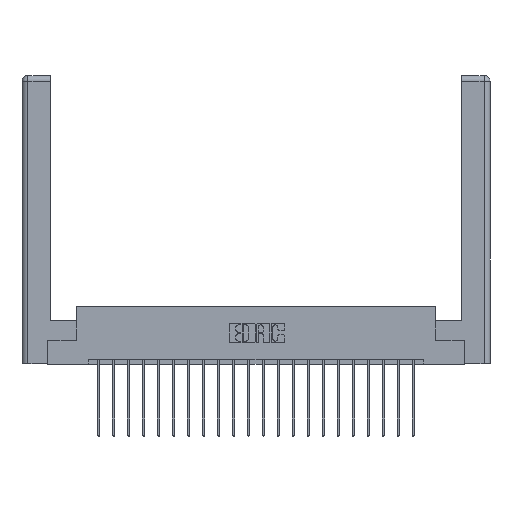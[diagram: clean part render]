
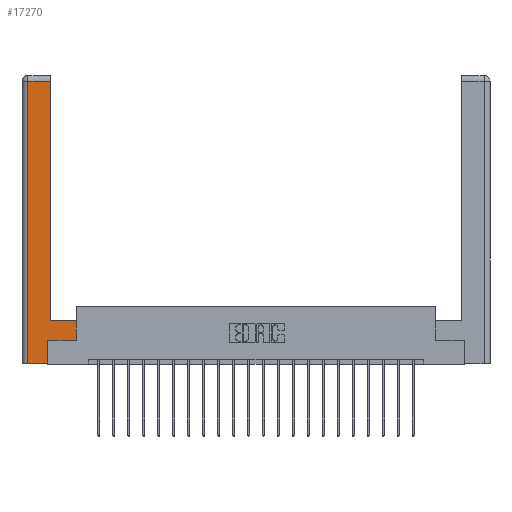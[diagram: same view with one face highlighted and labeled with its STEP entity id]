
A CAD part, top view. The second image highlights one B-rep face of the part: STEP entity #17270.
In plain terms, the highlighted planar face has unit normal (0, 0, 1).
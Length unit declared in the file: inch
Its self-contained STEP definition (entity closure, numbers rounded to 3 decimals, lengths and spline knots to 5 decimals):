
#39 = DIRECTION ( 'NONE',  ( 1., 0., 0. ) ) ;
#49 = CARTESIAN_POINT ( 'NONE',  ( 0.565, 0.245, 0. ) ) ;
#740 = DIRECTION ( 'NONE',  ( 0., 1., 0. ) ) ;
#1156 = AXIS2_PLACEMENT_3D ( 'NONE', #1345, #9943, #18810 ) ;
#1345 = CARTESIAN_POINT ( 'NONE',  ( 0., 0., 0. ) ) ;
#1348 = DIRECTION ( 'NONE',  ( 0., 1., 0. ) ) ;
#2506 = CARTESIAN_POINT ( 'NONE',  ( 0.265, 0.245, 0. ) ) ;
#2820 = EDGE_CURVE ( 'NONE', #22323, #15893, #14180, .T. ) ;
#3142 = VECTOR ( 'NONE', #3279, 39.37008 ) ;
#3279 = DIRECTION ( 'NONE',  ( 0., -1., 0. ) ) ;
#4844 = VERTEX_POINT ( 'NONE', #12020 ) ;
#5007 = CARTESIAN_POINT ( 'NONE',  ( 0.265, 0.245, 0. ) ) ;
#5040 = DIRECTION ( 'NONE',  ( -1., 0., 0. ) ) ;
#5057 = PLANE ( 'NONE',  #1156 ) ;
#5689 = EDGE_CURVE ( 'NONE', #21786, #22323, #20383, .T. ) ;
#5832 = ORIENTED_EDGE ( 'NONE', *, *, #7023, .T. ) ;
#6358 = DIRECTION ( 'NONE',  ( 1., 0., 0. ) ) ;
#7023 = EDGE_CURVE ( 'NONE', #4844, #11829, #10089, .T. ) ;
#7145 = CARTESIAN_POINT ( 'NONE',  ( 0.295, 0.45, 0. ) ) ;
#7484 = CARTESIAN_POINT ( 'NONE',  ( 0.0615, 2.94, 0. ) ) ;
#8630 = EDGE_CURVE ( 'NONE', #20529, #21786, #17831, .T. ) ;
#9102 = ORIENTED_EDGE ( 'NONE', *, *, #21248, .T. ) ;
#9279 = VECTOR ( 'NONE', #13780, 39.37008 ) ;
#9453 = ORIENTED_EDGE ( 'NONE', *, *, #16665, .T. ) ;
#9943 = DIRECTION ( 'NONE',  ( 0., 0., -1. ) ) ;
#10005 = ORIENTED_EDGE ( 'NONE', *, *, #2820, .T. ) ;
#10089 = LINE ( 'NONE', #7145, #9279 ) ;
#10149 = LINE ( 'NONE', #11698, #19314 ) ;
#10352 = VECTOR ( 'NONE', #740, 39.37008 ) ;
#10703 = ORIENTED_EDGE ( 'NONE', *, *, #5689, .T. ) ;
#11698 = CARTESIAN_POINT ( 'NONE',  ( 0.565, 0.45, 0. ) ) ;
#11829 = VERTEX_POINT ( 'NONE', #18217 ) ;
#11973 = CARTESIAN_POINT ( 'NONE',  ( 0.0615, 2.94, 0. ) ) ;
#12020 = CARTESIAN_POINT ( 'NONE',  ( 0.565, 0.45, 0. ) ) ;
#12190 = LINE ( 'NONE', #5007, #22132 ) ;
#12858 = ORIENTED_EDGE ( 'NONE', *, *, #14443, .T. ) ;
#13246 = VECTOR ( 'NONE', #5040, 39.37008 ) ;
#13780 = DIRECTION ( 'NONE',  ( -1., 0., 0. ) ) ;
#14180 = LINE ( 'NONE', #18865, #21970 ) ;
#14443 = EDGE_CURVE ( 'NONE', #11829, #20529, #17100, .T. ) ;
#14589 = CARTESIAN_POINT ( 'NONE',  ( 0.265, 0., 0. ) ) ;
#15084 = DIRECTION ( 'NONE',  ( 0., 1., 0. ) ) ;
#15893 = VERTEX_POINT ( 'NONE', #14589 ) ;
#16512 = CARTESIAN_POINT ( 'NONE',  ( 0.0615, 0., 0. ) ) ;
#16665 = EDGE_CURVE ( 'NONE', #15893, #18358, #12190, .T. ) ;
#17100 = LINE ( 'NONE', #21693, #10352 ) ;
#17270 = ADVANCED_FACE ( 'NONE', ( #18015 ), #5057, .F. ) ;
#17831 = LINE ( 'NONE', #11973, #13246 ) ;
#18015 = FACE_OUTER_BOUND ( 'NONE', #21316, .T. ) ;
#18217 = CARTESIAN_POINT ( 'NONE',  ( 0.295, 0.45, 0. ) ) ;
#18358 = VERTEX_POINT ( 'NONE', #2506 ) ;
#18577 = CARTESIAN_POINT ( 'NONE',  ( 0.565, 0.245, 0. ) ) ;
#18810 = DIRECTION ( 'NONE',  ( -1., 0., 0. ) ) ;
#18865 = CARTESIAN_POINT ( 'NONE',  ( 0.265, 0., 0. ) ) ;
#19028 = ORIENTED_EDGE ( 'NONE', *, *, #8630, .T. ) ;
#19314 = VECTOR ( 'NONE', #1348, 39.37008 ) ;
#19635 = LINE ( 'NONE', #18577, #21511 ) ;
#20383 = LINE ( 'NONE', #20597, #3142 ) ;
#20529 = VERTEX_POINT ( 'NONE', #21046 ) ;
#20597 = CARTESIAN_POINT ( 'NONE',  ( 0.0615, 0., 0. ) ) ;
#21046 = CARTESIAN_POINT ( 'NONE',  ( 0.295, 2.94, 0. ) ) ;
#21131 = ORIENTED_EDGE ( 'NONE', *, *, #21852, .T. ) ;
#21248 = EDGE_CURVE ( 'NONE', #18358, #21968, #19635, .T. ) ;
#21316 = EDGE_LOOP ( 'NONE', ( #12858, #19028, #10703, #10005, #9453, #9102, #21131, #5832 ) ) ;
#21511 = VECTOR ( 'NONE', #6358, 39.37008 ) ;
#21693 = CARTESIAN_POINT ( 'NONE',  ( 0.295, 3., 0. ) ) ;
#21786 = VERTEX_POINT ( 'NONE', #7484 ) ;
#21852 = EDGE_CURVE ( 'NONE', #21968, #4844, #10149, .T. ) ;
#21968 = VERTEX_POINT ( 'NONE', #49 ) ;
#21970 = VECTOR ( 'NONE', #39, 39.37008 ) ;
#22132 = VECTOR ( 'NONE', #15084, 39.37008 ) ;
#22323 = VERTEX_POINT ( 'NONE', #16512 ) ;
